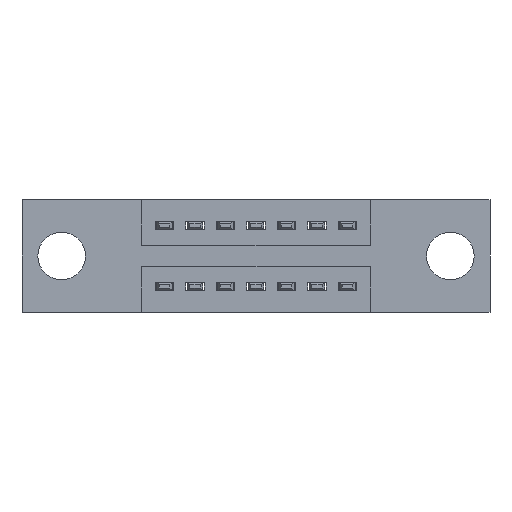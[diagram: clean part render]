
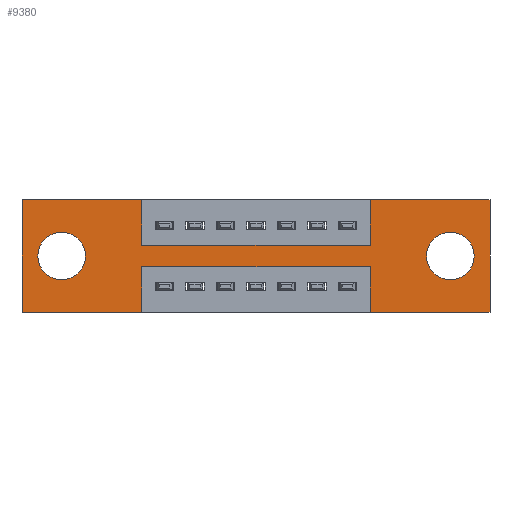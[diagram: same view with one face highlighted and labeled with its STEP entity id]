
A CAD part, front view. The second image highlights one B-rep face of the part: STEP entity #9380.
In plain terms, the highlighted planar face has unit normal (0, -1, 0).
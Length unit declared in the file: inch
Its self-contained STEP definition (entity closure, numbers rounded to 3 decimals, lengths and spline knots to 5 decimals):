
#40 = PLANE ( 'NONE',  #2962 ) ;
#161 = EDGE_CURVE ( 'NONE', #8738, #8171, #7540, .T. ) ;
#224 = VERTEX_POINT ( 'NONE', #8225 ) ;
#247 = AXIS2_PLACEMENT_3D ( 'NONE', #9544, #9543, #9531 ) ;
#357 = DIRECTION ( 'NONE',  ( -1., 0., 0. ) ) ;
#439 = CIRCLE ( 'NONE', #7428, 0.078 ) ;
#472 = VERTEX_POINT ( 'NONE', #2627 ) ;
#525 = CARTESIAN_POINT ( 'NONE',  ( 1.535, 0., 0. ) ) ;
#538 = ORIENTED_EDGE ( 'NONE', *, *, #5611, .F. ) ;
#585 = VERTEX_POINT ( 'NONE', #7602 ) ;
#702 = LINE ( 'NONE', #6947, #985 ) ;
#785 = FACE_BOUND ( 'NONE', #3640, .T. ) ;
#985 = VECTOR ( 'NONE', #7500, 39.37008 ) ;
#1057 = DIRECTION ( 'NONE',  ( 0., 0., -1. ) ) ;
#1068 = DIRECTION ( 'NONE',  ( 0., 1., 0. ) ) ;
#1078 = CARTESIAN_POINT ( 'NONE',  ( 1.405, 0., -0.185 ) ) ;
#1287 = CARTESIAN_POINT ( 'NONE',  ( 1.405, 0., -0.185 ) ) ;
#1447 = EDGE_CURVE ( 'NONE', #472, #9075, #9295, .T. ) ;
#1702 = CARTESIAN_POINT ( 'NONE',  ( 0.3925, 0., -0.22 ) ) ;
#1746 = DIRECTION ( 'NONE',  ( 0., 0., -1. ) ) ;
#1881 = VECTOR ( 'NONE', #8110, 39.37008 ) ;
#1944 = CARTESIAN_POINT ( 'NONE',  ( 0., 0., 0. ) ) ;
#1955 = CARTESIAN_POINT ( 'NONE',  ( 0.3925, 0., -0.15 ) ) ;
#2059 = LINE ( 'NONE', #4498, #9889 ) ;
#2127 = DIRECTION ( 'NONE',  ( 0., 0., -1. ) ) ;
#2390 = VERTEX_POINT ( 'NONE', #1955 ) ;
#2425 = EDGE_CURVE ( 'NONE', #2390, #8738, #7801, .T. ) ;
#2484 = CARTESIAN_POINT ( 'NONE',  ( 1.1425, 0., -0.37 ) ) ;
#2554 = EDGE_LOOP ( 'NONE', ( #3828, #4036 ) ) ;
#2627 = CARTESIAN_POINT ( 'NONE',  ( 1.535, 0., 0. ) ) ;
#2648 = CARTESIAN_POINT ( 'NONE',  ( 0.13, 0., -0.185 ) ) ;
#2776 = DIRECTION ( 'NONE',  ( 1., 0., 0. ) ) ;
#2867 = CIRCLE ( 'NONE', #247, 0.078 ) ;
#2884 = AXIS2_PLACEMENT_3D ( 'NONE', #2648, #7986, #3490 ) ;
#2962 = AXIS2_PLACEMENT_3D ( 'NONE', #5699, #6460, #1746 ) ;
#3130 = CARTESIAN_POINT ( 'NONE',  ( 1.1425, 0., -0.22 ) ) ;
#3173 = DIRECTION ( 'NONE',  ( -1., 0., 0. ) ) ;
#3284 = VECTOR ( 'NONE', #5621, 39.37008 ) ;
#3337 = VERTEX_POINT ( 'NONE', #9614 ) ;
#3340 = LINE ( 'NONE', #9086, #7137 ) ;
#3345 = EDGE_CURVE ( 'NONE', #7299, #224, #2867, .T. ) ;
#3490 = DIRECTION ( 'NONE',  ( 0., 0., 1. ) ) ;
#3545 = FACE_OUTER_BOUND ( 'NONE', #7917, .T. ) ;
#3576 = EDGE_CURVE ( 'NONE', #585, #3337, #8314, .T. ) ;
#3640 = EDGE_LOOP ( 'NONE', ( #4231, #5592 ) ) ;
#3703 = CARTESIAN_POINT ( 'NONE',  ( 1.1425, 0., 0. ) ) ;
#3828 = ORIENTED_EDGE ( 'NONE', *, *, #4936, .T. ) ;
#3934 = VERTEX_POINT ( 'NONE', #6249 ) ;
#4036 = ORIENTED_EDGE ( 'NONE', *, *, #9713, .T. ) ;
#4055 = DIRECTION ( 'NONE',  ( 0., 0., -1. ) ) ;
#4079 = LINE ( 'NONE', #1944, #7781 ) ;
#4223 = CARTESIAN_POINT ( 'NONE',  ( 0.3925, 0., -0.22 ) ) ;
#4231 = ORIENTED_EDGE ( 'NONE', *, *, #3345, .T. ) ;
#4262 = EDGE_CURVE ( 'NONE', #7440, #9079, #2059, .T. ) ;
#4443 = DIRECTION ( 'NONE',  ( 1., 0., 0. ) ) ;
#4498 = CARTESIAN_POINT ( 'NONE',  ( 0., 0., 0. ) ) ;
#4669 = CIRCLE ( 'NONE', #9012, 0.078 ) ;
#4670 = VECTOR ( 'NONE', #3173, 39.37008 ) ;
#4675 = CARTESIAN_POINT ( 'NONE',  ( 0.3925, 0., 0. ) ) ;
#4681 = CIRCLE ( 'NONE', #2884, 0.078 ) ;
#4936 = EDGE_CURVE ( 'NONE', #3934, #5333, #439, .T. ) ;
#5025 = CARTESIAN_POINT ( 'NONE',  ( 0.13, 0., -0.107 ) ) ;
#5272 = CARTESIAN_POINT ( 'NONE',  ( 0., 0., 0. ) ) ;
#5333 = VERTEX_POINT ( 'NONE', #9735 ) ;
#5368 = LINE ( 'NONE', #4223, #9045 ) ;
#5592 = ORIENTED_EDGE ( 'NONE', *, *, #7958, .T. ) ;
#5611 = EDGE_CURVE ( 'NONE', #3337, #7440, #3340, .T. ) ;
#5621 = DIRECTION ( 'NONE',  ( 0., 0., 1. ) ) ;
#5630 = VECTOR ( 'NONE', #4055, 39.37008 ) ;
#5699 = CARTESIAN_POINT ( 'NONE',  ( 0., 0., -0.37 ) ) ;
#5785 = EDGE_CURVE ( 'NONE', #9079, #2390, #7932, .T. ) ;
#5918 = EDGE_CURVE ( 'NONE', #7864, #585, #702, .T. ) ;
#6216 = VECTOR ( 'NONE', #7913, 39.37008 ) ;
#6249 = CARTESIAN_POINT ( 'NONE',  ( 1.405, 0., -0.107 ) ) ;
#6460 = DIRECTION ( 'NONE',  ( 0., -1., 0. ) ) ;
#6498 = CARTESIAN_POINT ( 'NONE',  ( 1.1425, 0., -0.15 ) ) ;
#6605 = EDGE_CURVE ( 'NONE', #9117, #7864, #5368, .T. ) ;
#6641 = VERTEX_POINT ( 'NONE', #9154 ) ;
#6650 = ORIENTED_EDGE ( 'NONE', *, *, #5918, .F. ) ;
#6754 = ORIENTED_EDGE ( 'NONE', *, *, #3576, .F. ) ;
#6798 = DIRECTION ( 'NONE',  ( 0., 1., 0. ) ) ;
#6847 = FACE_BOUND ( 'NONE', #2554, .T. ) ;
#6938 = ORIENTED_EDGE ( 'NONE', *, *, #6605, .F. ) ;
#6947 = CARTESIAN_POINT ( 'NONE',  ( 0.3925, 0., -0.37 ) ) ;
#6980 = CARTESIAN_POINT ( 'NONE',  ( 0., 0., -0.37 ) ) ;
#7116 = ORIENTED_EDGE ( 'NONE', *, *, #8561, .F. ) ;
#7137 = VECTOR ( 'NONE', #9119, 39.37008 ) ;
#7194 = ORIENTED_EDGE ( 'NONE', *, *, #8439, .F. ) ;
#7225 = ORIENTED_EDGE ( 'NONE', *, *, #1447, .F. ) ;
#7299 = VERTEX_POINT ( 'NONE', #5025 ) ;
#7346 = ORIENTED_EDGE ( 'NONE', *, *, #8815, .F. ) ;
#7365 = CARTESIAN_POINT ( 'NONE',  ( 0.3925, 0., -0.15 ) ) ;
#7428 = AXIS2_PLACEMENT_3D ( 'NONE', #1078, #1068, #1057 ) ;
#7440 = VERTEX_POINT ( 'NONE', #5272 ) ;
#7500 = DIRECTION ( 'NONE',  ( 0., 0., -1. ) ) ;
#7509 = ORIENTED_EDGE ( 'NONE', *, *, #161, .F. ) ;
#7540 = LINE ( 'NONE', #8130, #3284 ) ;
#7602 = CARTESIAN_POINT ( 'NONE',  ( 0.3925, 0., -0.37 ) ) ;
#7608 = CARTESIAN_POINT ( 'NONE',  ( 1.535, 0., -0.37 ) ) ;
#7658 = ORIENTED_EDGE ( 'NONE', *, *, #2425, .F. ) ;
#7668 = VECTOR ( 'NONE', #8541, 39.37008 ) ;
#7748 = ORIENTED_EDGE ( 'NONE', *, *, #5785, .F. ) ;
#7781 = VECTOR ( 'NONE', #2776, 39.37008 ) ;
#7801 = LINE ( 'NONE', #7365, #1881 ) ;
#7864 = VERTEX_POINT ( 'NONE', #1702 ) ;
#7875 = DIRECTION ( 'NONE',  ( -1., 0., 0. ) ) ;
#7903 = LINE ( 'NONE', #2484, #7668 ) ;
#7913 = DIRECTION ( 'NONE',  ( 0., 0., -1. ) ) ;
#7917 = EDGE_LOOP ( 'NONE', ( #6650, #6938, #7116, #7194, #7225, #7346, #7509, #7658, #7748, #8830, #538, #6754 ) ) ;
#7932 = LINE ( 'NONE', #8042, #6216 ) ;
#7958 = EDGE_CURVE ( 'NONE', #224, #7299, #4681, .T. ) ;
#7981 = CARTESIAN_POINT ( 'NONE',  ( 0., 0., -0.37 ) ) ;
#7986 = DIRECTION ( 'NONE',  ( 0., 1., 0. ) ) ;
#8042 = CARTESIAN_POINT ( 'NONE',  ( 0.3925, 0., 0. ) ) ;
#8097 = VECTOR ( 'NONE', #7875, 39.37008 ) ;
#8110 = DIRECTION ( 'NONE',  ( 1., 0., 0. ) ) ;
#8130 = CARTESIAN_POINT ( 'NONE',  ( 1.1425, 0., 0. ) ) ;
#8171 = VERTEX_POINT ( 'NONE', #3703 ) ;
#8225 = CARTESIAN_POINT ( 'NONE',  ( 0.13, 0., -0.263 ) ) ;
#8314 = LINE ( 'NONE', #7981, #8097 ) ;
#8439 = EDGE_CURVE ( 'NONE', #9075, #6641, #8588, .T. ) ;
#8541 = DIRECTION ( 'NONE',  ( 0., 0., 1. ) ) ;
#8561 = EDGE_CURVE ( 'NONE', #6641, #9117, #7903, .T. ) ;
#8588 = LINE ( 'NONE', #6980, #4670 ) ;
#8738 = VERTEX_POINT ( 'NONE', #6498 ) ;
#8815 = EDGE_CURVE ( 'NONE', #8171, #472, #4079, .T. ) ;
#8830 = ORIENTED_EDGE ( 'NONE', *, *, #4262, .F. ) ;
#9012 = AXIS2_PLACEMENT_3D ( 'NONE', #1287, #6798, #2127 ) ;
#9045 = VECTOR ( 'NONE', #357, 39.37008 ) ;
#9075 = VERTEX_POINT ( 'NONE', #7608 ) ;
#9079 = VERTEX_POINT ( 'NONE', #4675 ) ;
#9086 = CARTESIAN_POINT ( 'NONE',  ( 0., 0., 0. ) ) ;
#9117 = VERTEX_POINT ( 'NONE', #3130 ) ;
#9119 = DIRECTION ( 'NONE',  ( 0., 0., 1. ) ) ;
#9154 = CARTESIAN_POINT ( 'NONE',  ( 1.1425, 0., -0.37 ) ) ;
#9295 = LINE ( 'NONE', #525, #5630 ) ;
#9380 = ADVANCED_FACE ( 'NONE', ( #6847, #785, #3545 ), #40, .T. ) ;
#9531 = DIRECTION ( 'NONE',  ( 0., 0., 1. ) ) ;
#9543 = DIRECTION ( 'NONE',  ( 0., 1., 0. ) ) ;
#9544 = CARTESIAN_POINT ( 'NONE',  ( 0.13, 0., -0.185 ) ) ;
#9614 = CARTESIAN_POINT ( 'NONE',  ( 0., 0., -0.37 ) ) ;
#9713 = EDGE_CURVE ( 'NONE', #5333, #3934, #4669, .T. ) ;
#9735 = CARTESIAN_POINT ( 'NONE',  ( 1.405, 0., -0.263 ) ) ;
#9889 = VECTOR ( 'NONE', #4443, 39.37008 ) ;
